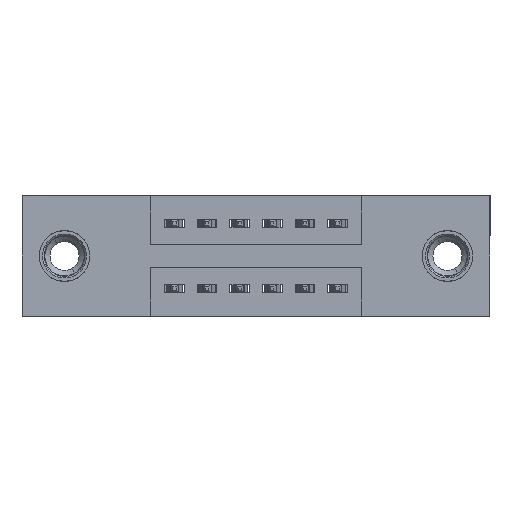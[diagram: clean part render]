
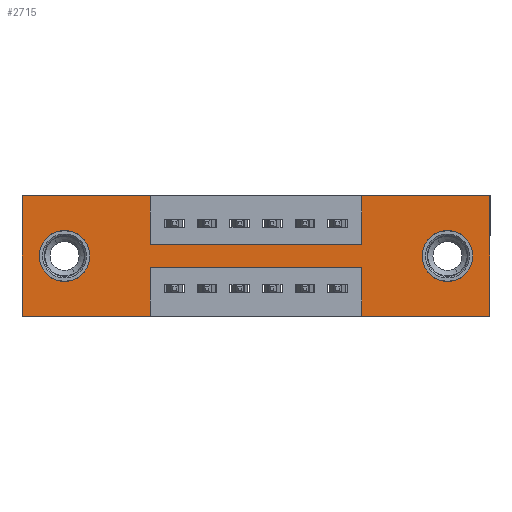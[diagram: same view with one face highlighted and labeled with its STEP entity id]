
A CAD part, front view. The second image highlights one B-rep face of the part: STEP entity #2715.
In plain terms, the highlighted planar face has unit normal (0, -1, 0).
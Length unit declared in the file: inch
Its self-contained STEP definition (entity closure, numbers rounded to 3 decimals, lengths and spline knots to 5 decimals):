
#247 = EDGE_CURVE ( 'NONE', #3055, #4077, #3447, .T. ) ;
#361 = CARTESIAN_POINT ( 'NONE',  ( 1.305, 0., -0.263 ) ) ;
#403 = VERTEX_POINT ( 'NONE', #5831 ) ;
#453 = CARTESIAN_POINT ( 'NONE',  ( 1.0425, 0., 0. ) ) ;
#454 = AXIS2_PLACEMENT_3D ( 'NONE', #12783, #10473, #13816 ) ;
#540 = CARTESIAN_POINT ( 'NONE',  ( 1.305, 0., -0.107 ) ) ;
#579 = AXIS2_PLACEMENT_3D ( 'NONE', #9520, #7255, #10489 ) ;
#868 = FACE_OUTER_BOUND ( 'NONE', #6688, .T. ) ;
#917 = ORIENTED_EDGE ( 'NONE', *, *, #14025, .F. ) ;
#953 = LINE ( 'NONE', #2831, #6743 ) ;
#957 = PLANE ( 'NONE',  #6503 ) ;
#1009 = CARTESIAN_POINT ( 'NONE',  ( 0., 0., -0.37 ) ) ;
#1043 = ORIENTED_EDGE ( 'NONE', *, *, #4055, .T. ) ;
#1085 = ORIENTED_EDGE ( 'NONE', *, *, #247, .F. ) ;
#1099 = DIRECTION ( 'NONE',  ( 0., 0., -1. ) ) ;
#1132 = VECTOR ( 'NONE', #9284, 39.37008 ) ;
#1348 = FACE_BOUND ( 'NONE', #6437, .T. ) ;
#1454 = CARTESIAN_POINT ( 'NONE',  ( 0., 0., 0. ) ) ;
#1578 = DIRECTION ( 'NONE',  ( 0., 0., -1. ) ) ;
#1605 = ORIENTED_EDGE ( 'NONE', *, *, #2113, .T. ) ;
#1618 = LINE ( 'NONE', #453, #1132 ) ;
#1703 = DIRECTION ( 'NONE',  ( 0., -1., 0. ) ) ;
#1823 = VECTOR ( 'NONE', #9477, 39.37008 ) ;
#2042 = ORIENTED_EDGE ( 'NONE', *, *, #12601, .F. ) ;
#2113 = EDGE_CURVE ( 'NONE', #14317, #4329, #10320, .T. ) ;
#2184 = EDGE_CURVE ( 'NONE', #12134, #13728, #9979, .T. ) ;
#2500 = VERTEX_POINT ( 'NONE', #1009 ) ;
#2715 = ADVANCED_FACE ( 'NONE', ( #7532, #1348, #868 ), #957, .T. ) ;
#2716 = DIRECTION ( 'NONE',  ( 1., 0., 0. ) ) ;
#2831 = CARTESIAN_POINT ( 'NONE',  ( 0.3925, 0., 0. ) ) ;
#2837 = CARTESIAN_POINT ( 'NONE',  ( 0.3925, 0., 0. ) ) ;
#3012 = ORIENTED_EDGE ( 'NONE', *, *, #2184, .T. ) ;
#3055 = VERTEX_POINT ( 'NONE', #7196 ) ;
#3084 = EDGE_CURVE ( 'NONE', #13728, #12134, #10294, .T. ) ;
#3242 = CARTESIAN_POINT ( 'NONE',  ( 0.13, 0., -0.107 ) ) ;
#3447 = LINE ( 'NONE', #6521, #5473 ) ;
#3495 = CARTESIAN_POINT ( 'NONE',  ( 0., 0., 0. ) ) ;
#3746 = CARTESIAN_POINT ( 'NONE',  ( 0., 0., -0.37 ) ) ;
#3818 = CARTESIAN_POINT ( 'NONE',  ( 0., 0., 0. ) ) ;
#3998 = CARTESIAN_POINT ( 'NONE',  ( 0.3925, 0., -0.37 ) ) ;
#4055 = EDGE_CURVE ( 'NONE', #4329, #14317, #13416, .T. ) ;
#4077 = VERTEX_POINT ( 'NONE', #4106 ) ;
#4106 = CARTESIAN_POINT ( 'NONE',  ( 1.435, 0., 0. ) ) ;
#4154 = CARTESIAN_POINT ( 'NONE',  ( 1.305, 0., -0.185 ) ) ;
#4165 = DIRECTION ( 'NONE',  ( 0., 0., -1. ) ) ;
#4328 = AXIS2_PLACEMENT_3D ( 'NONE', #7949, #11454, #1578 ) ;
#4329 = VERTEX_POINT ( 'NONE', #361 ) ;
#4377 = EDGE_CURVE ( 'NONE', #12232, #9097, #13400, .T. ) ;
#4470 = DIRECTION ( 'NONE',  ( 1., 0., 0. ) ) ;
#4868 = CARTESIAN_POINT ( 'NONE',  ( 0., 0., -0.37 ) ) ;
#4946 = CARTESIAN_POINT ( 'NONE',  ( 0., 0., -0.37 ) ) ;
#5195 = DIRECTION ( 'NONE',  ( 0., 0., -1. ) ) ;
#5217 = EDGE_CURVE ( 'NONE', #4077, #12232, #10954, .T. ) ;
#5473 = VECTOR ( 'NONE', #4470, 39.37008 ) ;
#5507 = EDGE_CURVE ( 'NONE', #11278, #2500, #7801, .T. ) ;
#5701 = ORIENTED_EDGE ( 'NONE', *, *, #5993, .F. ) ;
#5747 = EDGE_CURVE ( 'NONE', #7693, #9337, #953, .T. ) ;
#5831 = CARTESIAN_POINT ( 'NONE',  ( 0.3925, 0., -0.22 ) ) ;
#5993 = EDGE_CURVE ( 'NONE', #7566, #403, #13366, .T. ) ;
#6046 = EDGE_CURVE ( 'NONE', #9097, #7566, #13717, .T. ) ;
#6356 = LINE ( 'NONE', #3818, #13857 ) ;
#6437 = EDGE_LOOP ( 'NONE', ( #3012, #14255 ) ) ;
#6447 = VECTOR ( 'NONE', #10635, 39.37008 ) ;
#6503 = AXIS2_PLACEMENT_3D ( 'NONE', #4946, #1703, #4165 ) ;
#6521 = CARTESIAN_POINT ( 'NONE',  ( 0., 0., 0. ) ) ;
#6605 = CARTESIAN_POINT ( 'NONE',  ( 0.3925, 0., -0.37 ) ) ;
#6688 = EDGE_LOOP ( 'NONE', ( #11704, #5701, #11803, #8650, #8676, #1085, #13598, #917, #8858, #8625, #2042, #12540 ) ) ;
#6703 = CARTESIAN_POINT ( 'NONE',  ( 0.3925, 0., -0.22 ) ) ;
#6743 = VECTOR ( 'NONE', #10506, 39.37008 ) ;
#6899 = VECTOR ( 'NONE', #7959, 39.37008 ) ;
#6971 = VERTEX_POINT ( 'NONE', #7709 ) ;
#7028 = CARTESIAN_POINT ( 'NONE',  ( 0.13, 0., -0.263 ) ) ;
#7196 = CARTESIAN_POINT ( 'NONE',  ( 1.0425, 0., 0. ) ) ;
#7244 = CARTESIAN_POINT ( 'NONE',  ( 1.0425, 0., -0.22 ) ) ;
#7255 = DIRECTION ( 'NONE',  ( 0., 1., 0. ) ) ;
#7431 = LINE ( 'NONE', #6605, #13336 ) ;
#7532 = FACE_BOUND ( 'NONE', #11626, .T. ) ;
#7566 = VERTEX_POINT ( 'NONE', #7244 ) ;
#7693 = VERTEX_POINT ( 'NONE', #2837 ) ;
#7709 = CARTESIAN_POINT ( 'NONE',  ( 1.0425, 0., -0.15 ) ) ;
#7801 = LINE ( 'NONE', #4868, #9734 ) ;
#7949 = CARTESIAN_POINT ( 'NONE',  ( 1.305, 0., -0.185 ) ) ;
#7959 = DIRECTION ( 'NONE',  ( 0., 0., 1. ) ) ;
#8311 = EDGE_CURVE ( 'NONE', #12966, #7693, #6356, .T. ) ;
#8625 = ORIENTED_EDGE ( 'NONE', *, *, #8311, .F. ) ;
#8650 = ORIENTED_EDGE ( 'NONE', *, *, #4377, .F. ) ;
#8676 = ORIENTED_EDGE ( 'NONE', *, *, #5217, .F. ) ;
#8858 = ORIENTED_EDGE ( 'NONE', *, *, #5747, .F. ) ;
#9003 = DIRECTION ( 'NONE',  ( 0., 0., 1. ) ) ;
#9097 = VERTEX_POINT ( 'NONE', #12685 ) ;
#9284 = DIRECTION ( 'NONE',  ( 0., 0., 1. ) ) ;
#9319 = EDGE_CURVE ( 'NONE', #6971, #3055, #1618, .T. ) ;
#9337 = VERTEX_POINT ( 'NONE', #12730 ) ;
#9477 = DIRECTION ( 'NONE',  ( 0., 0., -1. ) ) ;
#9520 = CARTESIAN_POINT ( 'NONE',  ( 0.13, 0., -0.185 ) ) ;
#9734 = VECTOR ( 'NONE', #13976, 39.37008 ) ;
#9950 = LINE ( 'NONE', #12992, #6447 ) ;
#9969 = DIRECTION ( 'NONE',  ( -1., 0., 0. ) ) ;
#9979 = CIRCLE ( 'NONE', #454, 0.078 ) ;
#9982 = LINE ( 'NONE', #3495, #11546 ) ;
#10147 = AXIS2_PLACEMENT_3D ( 'NONE', #4154, #14098, #5195 ) ;
#10293 = CARTESIAN_POINT ( 'NONE',  ( 1.0425, 0., -0.37 ) ) ;
#10294 = CIRCLE ( 'NONE', #579, 0.078 ) ;
#10320 = CIRCLE ( 'NONE', #4328, 0.078 ) ;
#10418 = EDGE_CURVE ( 'NONE', #403, #11278, #7431, .T. ) ;
#10473 = DIRECTION ( 'NONE',  ( 0., 1., 0. ) ) ;
#10489 = DIRECTION ( 'NONE',  ( 0., 0., 1. ) ) ;
#10506 = DIRECTION ( 'NONE',  ( 0., 0., -1. ) ) ;
#10556 = CARTESIAN_POINT ( 'NONE',  ( 1.435, 0., 0. ) ) ;
#10635 = DIRECTION ( 'NONE',  ( 1., 0., 0. ) ) ;
#10954 = LINE ( 'NONE', #10556, #1823 ) ;
#11278 = VERTEX_POINT ( 'NONE', #3998 ) ;
#11454 = DIRECTION ( 'NONE',  ( 0., 1., 0. ) ) ;
#11464 = DIRECTION ( 'NONE',  ( -1., 0., 0. ) ) ;
#11546 = VECTOR ( 'NONE', #9003, 39.37008 ) ;
#11626 = EDGE_LOOP ( 'NONE', ( #1605, #1043 ) ) ;
#11704 = ORIENTED_EDGE ( 'NONE', *, *, #10418, .F. ) ;
#11803 = ORIENTED_EDGE ( 'NONE', *, *, #6046, .F. ) ;
#11818 = VECTOR ( 'NONE', #9969, 39.37008 ) ;
#12134 = VERTEX_POINT ( 'NONE', #3242 ) ;
#12202 = VECTOR ( 'NONE', #11464, 39.37008 ) ;
#12232 = VERTEX_POINT ( 'NONE', #12698 ) ;
#12540 = ORIENTED_EDGE ( 'NONE', *, *, #5507, .F. ) ;
#12601 = EDGE_CURVE ( 'NONE', #2500, #12966, #9982, .T. ) ;
#12685 = CARTESIAN_POINT ( 'NONE',  ( 1.0425, 0., -0.37 ) ) ;
#12698 = CARTESIAN_POINT ( 'NONE',  ( 1.435, 0., -0.37 ) ) ;
#12730 = CARTESIAN_POINT ( 'NONE',  ( 0.3925, 0., -0.15 ) ) ;
#12783 = CARTESIAN_POINT ( 'NONE',  ( 0.13, 0., -0.185 ) ) ;
#12966 = VERTEX_POINT ( 'NONE', #1454 ) ;
#12992 = CARTESIAN_POINT ( 'NONE',  ( 0.3925, 0., -0.15 ) ) ;
#13336 = VECTOR ( 'NONE', #1099, 39.37008 ) ;
#13366 = LINE ( 'NONE', #6703, #11818 ) ;
#13400 = LINE ( 'NONE', #3746, #12202 ) ;
#13416 = CIRCLE ( 'NONE', #10147, 0.078 ) ;
#13598 = ORIENTED_EDGE ( 'NONE', *, *, #9319, .F. ) ;
#13717 = LINE ( 'NONE', #10293, #6899 ) ;
#13728 = VERTEX_POINT ( 'NONE', #7028 ) ;
#13816 = DIRECTION ( 'NONE',  ( 0., 0., 1. ) ) ;
#13857 = VECTOR ( 'NONE', #2716, 39.37008 ) ;
#13976 = DIRECTION ( 'NONE',  ( -1., 0., 0. ) ) ;
#14025 = EDGE_CURVE ( 'NONE', #9337, #6971, #9950, .T. ) ;
#14098 = DIRECTION ( 'NONE',  ( 0., 1., 0. ) ) ;
#14255 = ORIENTED_EDGE ( 'NONE', *, *, #3084, .T. ) ;
#14317 = VERTEX_POINT ( 'NONE', #540 ) ;
